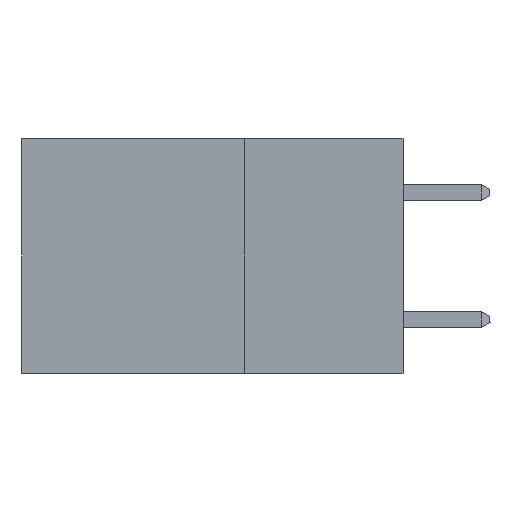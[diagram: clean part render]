
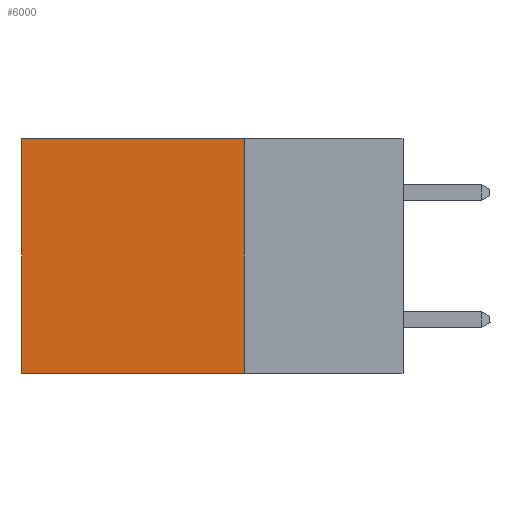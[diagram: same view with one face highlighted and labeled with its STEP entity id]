
A CAD part, left-side view. The second image highlights one B-rep face of the part: STEP entity #6000.
In plain terms, the highlighted planar face has unit normal (-1, 0, 0).
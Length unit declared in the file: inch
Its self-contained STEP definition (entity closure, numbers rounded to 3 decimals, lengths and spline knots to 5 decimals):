
#271 = EDGE_CURVE ( 'NONE', #8602, #10102, #5985, .T. ) ;
#925 = CARTESIAN_POINT ( 'NONE',  ( 0.2875, 0.25, 0. ) ) ;
#1245 = DIRECTION ( 'NONE',  ( 0., 1., 0. ) ) ;
#1316 = ORIENTED_EDGE ( 'NONE', *, *, #271, .F. ) ;
#1859 = VECTOR ( 'NONE', #1245, 39.37008 ) ;
#3142 = DIRECTION ( 'NONE',  ( 0., 0., -1. ) ) ;
#3239 = EDGE_CURVE ( 'NONE', #8602, #3838, #4782, .T. ) ;
#3400 = CARTESIAN_POINT ( 'NONE',  ( 0.2875, 0.25, 0. ) ) ;
#3661 = ORIENTED_EDGE ( 'NONE', *, *, #3239, .T. ) ;
#3793 = DIRECTION ( 'NONE',  ( 0., 1., 0. ) ) ;
#3838 = VERTEX_POINT ( 'NONE', #8565 ) ;
#4021 = LINE ( 'NONE', #10277, #12938 ) ;
#4692 = LINE ( 'NONE', #5060, #12944 ) ;
#4782 = LINE ( 'NONE', #3400, #1859 ) ;
#5060 = CARTESIAN_POINT ( 'NONE',  ( 0.2875, 0.6, 0. ) ) ;
#5640 = VECTOR ( 'NONE', #12479, 39.37008 ) ;
#5985 = LINE ( 'NONE', #12768, #5640 ) ;
#6000 = ADVANCED_FACE ( 'NONE', ( #8121 ), #9633, .F. ) ;
#6286 = CARTESIAN_POINT ( 'NONE',  ( 0.2875, 0.6, -0.37 ) ) ;
#7153 = EDGE_CURVE ( 'NONE', #3838, #13127, #4692, .T. ) ;
#8121 = FACE_OUTER_BOUND ( 'NONE', #9037, .T. ) ;
#8565 = CARTESIAN_POINT ( 'NONE',  ( 0.2875, 0.6, 0. ) ) ;
#8602 = VERTEX_POINT ( 'NONE', #10797 ) ;
#8802 = AXIS2_PLACEMENT_3D ( 'NONE', #925, #12798, #3142 ) ;
#9037 = EDGE_LOOP ( 'NONE', ( #9563, #11115, #1316, #3661 ) ) ;
#9563 = ORIENTED_EDGE ( 'NONE', *, *, #7153, .T. ) ;
#9633 = PLANE ( 'NONE',  #8802 ) ;
#10102 = VERTEX_POINT ( 'NONE', #10338 ) ;
#10277 = CARTESIAN_POINT ( 'NONE',  ( 0.2875, 0.25, -0.37 ) ) ;
#10338 = CARTESIAN_POINT ( 'NONE',  ( 0.2875, 0.25, -0.37 ) ) ;
#10460 = DIRECTION ( 'NONE',  ( 0., 0., -1. ) ) ;
#10668 = EDGE_CURVE ( 'NONE', #10102, #13127, #4021, .T. ) ;
#10797 = CARTESIAN_POINT ( 'NONE',  ( 0.2875, 0.25, 0. ) ) ;
#11115 = ORIENTED_EDGE ( 'NONE', *, *, #10668, .F. ) ;
#12479 = DIRECTION ( 'NONE',  ( 0., 0., -1. ) ) ;
#12768 = CARTESIAN_POINT ( 'NONE',  ( 0.2875, 0.25, 0. ) ) ;
#12798 = DIRECTION ( 'NONE',  ( 1., 0., 0. ) ) ;
#12938 = VECTOR ( 'NONE', #3793, 39.37008 ) ;
#12944 = VECTOR ( 'NONE', #10460, 39.37008 ) ;
#13127 = VERTEX_POINT ( 'NONE', #6286 ) ;
